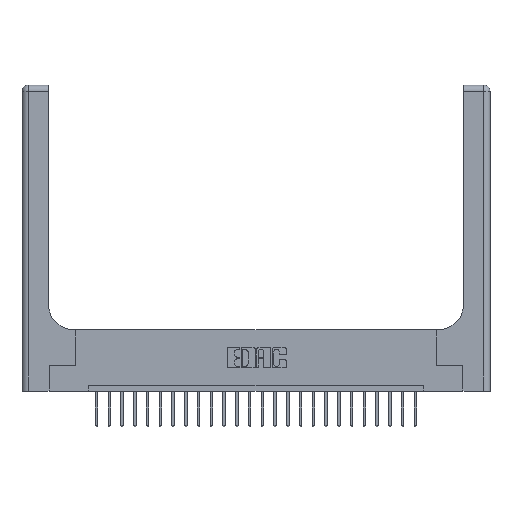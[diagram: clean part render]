
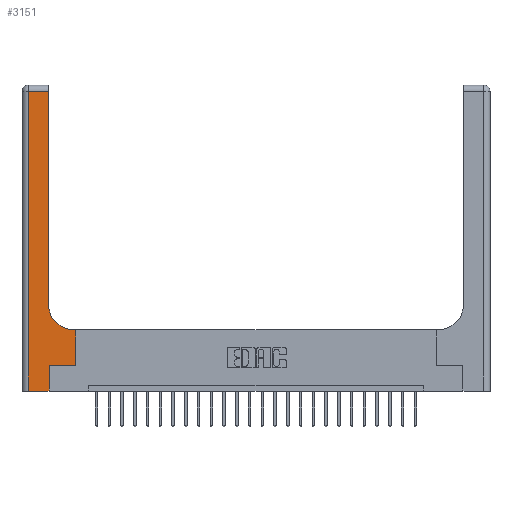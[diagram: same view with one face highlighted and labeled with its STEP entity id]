
A CAD part, top view. The second image highlights one B-rep face of the part: STEP entity #3151.
In plain terms, the highlighted planar face has unit normal (0, 0, 1).
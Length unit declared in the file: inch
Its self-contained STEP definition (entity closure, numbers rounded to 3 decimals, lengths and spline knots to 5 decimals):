
#277 = CARTESIAN_POINT ( 'NONE',  ( 0.265, 0., 0.37 ) ) ;
#532 = ORIENTED_EDGE ( 'NONE', *, *, #21223, .T. ) ;
#909 = CARTESIAN_POINT ( 'NONE',  ( 0., 2.94, 0.37 ) ) ;
#1233 = EDGE_CURVE ( 'NONE', #18358, #13684, #19598, .T. ) ;
#1646 = VERTEX_POINT ( 'NONE', #20613 ) ;
#1840 = DIRECTION ( 'NONE',  ( 1., 0., 0. ) ) ;
#2365 = VECTOR ( 'NONE', #19030, 39.37008 ) ;
#2997 = CARTESIAN_POINT ( 'NONE',  ( 0.528, 0.25, 0.37 ) ) ;
#3014 = DIRECTION ( 'NONE',  ( 0., 1., 0. ) ) ;
#3085 = EDGE_CURVE ( 'NONE', #13684, #9764, #16160, .T. ) ;
#3087 = DIRECTION ( 'NONE',  ( 1., 0., 0. ) ) ;
#3105 = VERTEX_POINT ( 'NONE', #19414 ) ;
#3151 = ADVANCED_FACE ( 'NONE', ( #16874 ), #3441, .F. ) ;
#3234 = AXIS2_PLACEMENT_3D ( 'NONE', #8797, #23662, #3087 ) ;
#3441 = PLANE ( 'NONE',  #7061 ) ;
#3593 = LINE ( 'NONE', #11123, #10655 ) ;
#4618 = CARTESIAN_POINT ( 'NONE',  ( 0.26, 3., 0.37 ) ) ;
#4649 = VERTEX_POINT ( 'NONE', #9958 ) ;
#4722 = VECTOR ( 'NONE', #1840, 39.37008 ) ;
#5219 = EDGE_CURVE ( 'NONE', #15436, #3105, #3593, .T. ) ;
#5532 = CARTESIAN_POINT ( 'NONE',  ( 0.528, 0.6, 0.37 ) ) ;
#5882 = VECTOR ( 'NONE', #3014, 39.37008 ) ;
#6632 = CARTESIAN_POINT ( 'NONE',  ( 0.06, 2.94, 0.37 ) ) ;
#6704 = VECTOR ( 'NONE', #23231, 39.37008 ) ;
#7061 = AXIS2_PLACEMENT_3D ( 'NONE', #20264, #20384, #22176 ) ;
#7342 = EDGE_CURVE ( 'NONE', #3105, #4649, #22279, .T. ) ;
#7461 = ORIENTED_EDGE ( 'NONE', *, *, #3085, .T. ) ;
#7558 = CARTESIAN_POINT ( 'NONE',  ( 0.265, 0.25, 0.37 ) ) ;
#8317 = LINE ( 'NONE', #909, #22654 ) ;
#8797 = CARTESIAN_POINT ( 'NONE',  ( 0.51, 0.85, 0.37 ) ) ;
#9644 = EDGE_CURVE ( 'NONE', #21708, #1646, #20940, .T. ) ;
#9764 = VERTEX_POINT ( 'NONE', #15986 ) ;
#9958 = CARTESIAN_POINT ( 'NONE',  ( 0.265, 0., 0.37 ) ) ;
#10442 = EDGE_CURVE ( 'NONE', #9764, #21708, #14071, .T. ) ;
#10476 = ORIENTED_EDGE ( 'NONE', *, *, #15588, .T. ) ;
#10655 = VECTOR ( 'NONE', #22090, 39.37008 ) ;
#10860 = ORIENTED_EDGE ( 'NONE', *, *, #7342, .T. ) ;
#11073 = CARTESIAN_POINT ( 'NONE',  ( 0., 0., 0.37 ) ) ;
#11123 = CARTESIAN_POINT ( 'NONE',  ( 0.06, 3., 0.37 ) ) ;
#11929 = CARTESIAN_POINT ( 'NONE',  ( 0.26, 0.85, 0.37 ) ) ;
#12328 = ORIENTED_EDGE ( 'NONE', *, *, #9644, .T. ) ;
#13230 = VECTOR ( 'NONE', #18096, 39.37008 ) ;
#13684 = VERTEX_POINT ( 'NONE', #5532 ) ;
#14071 = CIRCLE ( 'NONE', #3234, 0.25 ) ;
#14338 = CARTESIAN_POINT ( 'NONE',  ( 0.26, 0.6, 0.37 ) ) ;
#14400 = CARTESIAN_POINT ( 'NONE',  ( 0.528, 0.25, 0.37 ) ) ;
#15436 = VERTEX_POINT ( 'NONE', #6632 ) ;
#15550 = EDGE_CURVE ( 'NONE', #21888, #18358, #19144, .T. ) ;
#15588 = EDGE_CURVE ( 'NONE', #4649, #21888, #16866, .T. ) ;
#15986 = CARTESIAN_POINT ( 'NONE',  ( 0.51, 0.6, 0.37 ) ) ;
#16160 = LINE ( 'NONE', #14338, #13230 ) ;
#16393 = EDGE_LOOP ( 'NONE', ( #12328, #532, #22726, #10860, #10476, #20142, #23826, #7461, #20027 ) ) ;
#16866 = LINE ( 'NONE', #277, #23624 ) ;
#16874 = FACE_OUTER_BOUND ( 'NONE', #16393, .T. ) ;
#18096 = DIRECTION ( 'NONE',  ( -1., 0., 0. ) ) ;
#18358 = VERTEX_POINT ( 'NONE', #2997 ) ;
#18846 = DIRECTION ( 'NONE',  ( -1., 0., 0. ) ) ;
#19030 = DIRECTION ( 'NONE',  ( 1., 0., 0. ) ) ;
#19144 = LINE ( 'NONE', #7558, #2365 ) ;
#19414 = CARTESIAN_POINT ( 'NONE',  ( 0.06, 0., 0.37 ) ) ;
#19598 = LINE ( 'NONE', #14400, #5882 ) ;
#20027 = ORIENTED_EDGE ( 'NONE', *, *, #10442, .T. ) ;
#20142 = ORIENTED_EDGE ( 'NONE', *, *, #15550, .T. ) ;
#20264 = CARTESIAN_POINT ( 'NONE',  ( 0., 3., 0.37 ) ) ;
#20384 = DIRECTION ( 'NONE',  ( 0., 0., -1. ) ) ;
#20488 = DIRECTION ( 'NONE',  ( 0., 1., 0. ) ) ;
#20613 = CARTESIAN_POINT ( 'NONE',  ( 0.26, 2.94, 0.37 ) ) ;
#20940 = LINE ( 'NONE', #4618, #6704 ) ;
#21223 = EDGE_CURVE ( 'NONE', #1646, #15436, #8317, .T. ) ;
#21580 = CARTESIAN_POINT ( 'NONE',  ( 0.265, 0.25, 0.37 ) ) ;
#21708 = VERTEX_POINT ( 'NONE', #11929 ) ;
#21888 = VERTEX_POINT ( 'NONE', #21580 ) ;
#22090 = DIRECTION ( 'NONE',  ( 0., -1., 0. ) ) ;
#22176 = DIRECTION ( 'NONE',  ( -1., 0., 0. ) ) ;
#22279 = LINE ( 'NONE', #11073, #4722 ) ;
#22654 = VECTOR ( 'NONE', #18846, 39.37008 ) ;
#22726 = ORIENTED_EDGE ( 'NONE', *, *, #5219, .T. ) ;
#23231 = DIRECTION ( 'NONE',  ( 0., 1., 0. ) ) ;
#23624 = VECTOR ( 'NONE', #20488, 39.37008 ) ;
#23662 = DIRECTION ( 'NONE',  ( 0., 0., -1. ) ) ;
#23826 = ORIENTED_EDGE ( 'NONE', *, *, #1233, .T. ) ;
